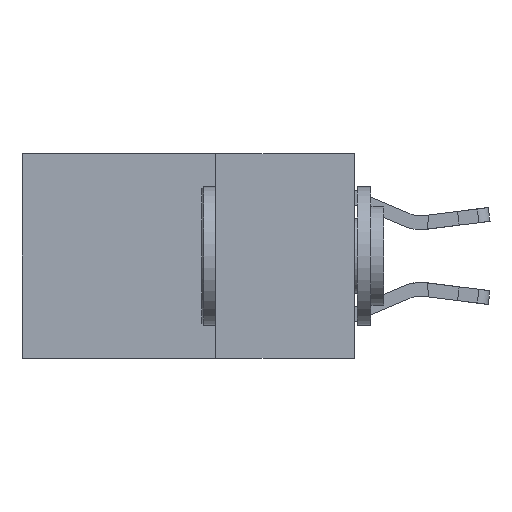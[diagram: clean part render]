
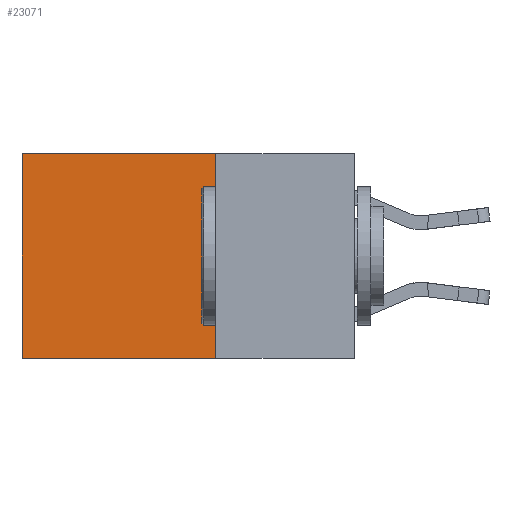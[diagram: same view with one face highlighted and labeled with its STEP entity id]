
A CAD part, left-side view. The second image highlights one B-rep face of the part: STEP entity #23071.
In plain terms, the highlighted planar face has unit normal (-1, 0, 0).
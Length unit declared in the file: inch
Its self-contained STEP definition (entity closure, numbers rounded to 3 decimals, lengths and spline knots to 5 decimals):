
#792 = AXIS2_PLACEMENT_3D ( 'NONE', #12012, #15719, #17620 ) ;
#1320 = VECTOR ( 'NONE', #21616, 39.37008 ) ;
#1581 = EDGE_CURVE ( 'NONE', #7185, #20167, #18395, .T. ) ;
#1621 = CARTESIAN_POINT ( 'NONE',  ( 0.2625, 0.6, 0. ) ) ;
#2104 = EDGE_CURVE ( 'NONE', #17450, #7185, #9846, .T. ) ;
#2188 = CARTESIAN_POINT ( 'NONE',  ( 0.2625, 0.25, 0. ) ) ;
#2475 = EDGE_LOOP ( 'NONE', ( #12902, #8873, #12647, #13175 ) ) ;
#2799 = FACE_OUTER_BOUND ( 'NONE', #2475, .T. ) ;
#5099 = CARTESIAN_POINT ( 'NONE',  ( 0.2625, 0.25, 0. ) ) ;
#5643 = EDGE_CURVE ( 'NONE', #15422, #20167, #6917, .T. ) ;
#6917 = LINE ( 'NONE', #10376, #1320 ) ;
#7011 = LINE ( 'NONE', #5099, #12541 ) ;
#7185 = VERTEX_POINT ( 'NONE', #22926 ) ;
#7264 = EDGE_CURVE ( 'NONE', #17450, #15422, #7011, .T. ) ;
#8873 = ORIENTED_EDGE ( 'NONE', *, *, #1581, .F. ) ;
#9476 = VECTOR ( 'NONE', #20607, 39.37008 ) ;
#9846 = LINE ( 'NONE', #9962, #9476 ) ;
#9962 = CARTESIAN_POINT ( 'NONE',  ( 0.2625, 0.25, 0. ) ) ;
#10376 = CARTESIAN_POINT ( 'NONE',  ( 0.2625, 0.6, 0. ) ) ;
#12012 = CARTESIAN_POINT ( 'NONE',  ( 0.2625, 0.25, 0. ) ) ;
#12541 = VECTOR ( 'NONE', #14088, 39.37008 ) ;
#12647 = ORIENTED_EDGE ( 'NONE', *, *, #2104, .F. ) ;
#12902 = ORIENTED_EDGE ( 'NONE', *, *, #5643, .T. ) ;
#13175 = ORIENTED_EDGE ( 'NONE', *, *, #7264, .T. ) ;
#14088 = DIRECTION ( 'NONE',  ( 0., 1., 0. ) ) ;
#15422 = VERTEX_POINT ( 'NONE', #1621 ) ;
#15719 = DIRECTION ( 'NONE',  ( 1., 0., 0. ) ) ;
#17450 = VERTEX_POINT ( 'NONE', #2188 ) ;
#17620 = DIRECTION ( 'NONE',  ( 0., 0., -1. ) ) ;
#18395 = LINE ( 'NONE', #21994, #22428 ) ;
#19053 = PLANE ( 'NONE',  #792 ) ;
#19724 = DIRECTION ( 'NONE',  ( 0., 1., 0. ) ) ;
#20167 = VERTEX_POINT ( 'NONE', #22288 ) ;
#20607 = DIRECTION ( 'NONE',  ( 0., 0., -1. ) ) ;
#21616 = DIRECTION ( 'NONE',  ( 0., 0., -1. ) ) ;
#21994 = CARTESIAN_POINT ( 'NONE',  ( 0.2625, 0.25, -0.37 ) ) ;
#22288 = CARTESIAN_POINT ( 'NONE',  ( 0.2625, 0.6, -0.37 ) ) ;
#22428 = VECTOR ( 'NONE', #19724, 39.37008 ) ;
#22926 = CARTESIAN_POINT ( 'NONE',  ( 0.2625, 0.25, -0.37 ) ) ;
#23071 = ADVANCED_FACE ( 'NONE', ( #2799 ), #19053, .F. ) ;
